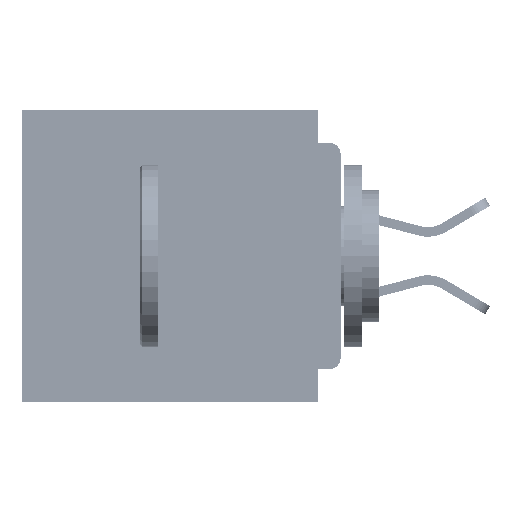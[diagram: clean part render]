
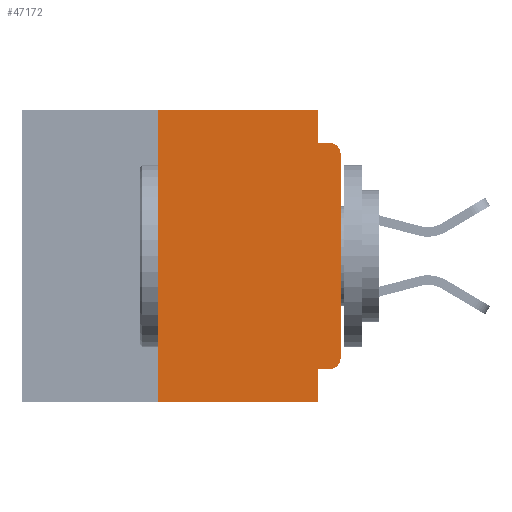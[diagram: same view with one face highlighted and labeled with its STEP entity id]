
A CAD part, left-side view. The second image highlights one B-rep face of the part: STEP entity #47172.
In plain terms, the highlighted planar face has unit normal (-1, 0, 0).
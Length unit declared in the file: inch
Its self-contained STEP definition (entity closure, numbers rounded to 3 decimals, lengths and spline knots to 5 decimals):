
#32 = CARTESIAN_POINT ( 'NONE',  ( 0., 0.25, -0.4 ) ) ;
#1003 = CARTESIAN_POINT ( 'NONE',  ( 0., 0., -0.355 ) ) ;
#1164 = VECTOR ( 'NONE', #13344, 39.37008 ) ;
#1187 = LINE ( 'NONE', #27473, #43794 ) ;
#1316 = CARTESIAN_POINT ( 'NONE',  ( 0., 0.031, 0. ) ) ;
#1366 = DIRECTION ( 'NONE',  ( 0., 0., -1. ) ) ;
#1880 = VECTOR ( 'NONE', #17656, 39.37008 ) ;
#2666 = VECTOR ( 'NONE', #46328, 39.37008 ) ;
#2784 = EDGE_CURVE ( 'NONE', #44498, #15873, #3217, .T. ) ;
#3217 = LINE ( 'NONE', #53201, #23938 ) ;
#3515 = VERTEX_POINT ( 'NONE', #24632 ) ;
#3997 = EDGE_CURVE ( 'NONE', #20755, #44498, #15372, .T. ) ;
#4605 = ORIENTED_EDGE ( 'NONE', *, *, #16691, .T. ) ;
#5073 = DIRECTION ( 'NONE',  ( 0., 0., 1. ) ) ;
#5214 = DIRECTION ( 'NONE',  ( 1., 0., 0. ) ) ;
#5673 = LINE ( 'NONE', #50269, #1164 ) ;
#8948 = CARTESIAN_POINT ( 'NONE',  ( 0., 0.031, -0.045 ) ) ;
#9194 = CARTESIAN_POINT ( 'NONE',  ( 0., 0.015, -0.045 ) ) ;
#9351 = EDGE_CURVE ( 'NONE', #37884, #3515, #34268, .T. ) ;
#9476 = ORIENTED_EDGE ( 'NONE', *, *, #37555, .T. ) ;
#9856 = CIRCLE ( 'NONE', #25262, 0.015 ) ;
#9938 = AXIS2_PLACEMENT_3D ( 'NONE', #29965, #5214, #34076 ) ;
#10541 = EDGE_CURVE ( 'NONE', #29381, #37884, #34785, .T. ) ;
#10884 = ORIENTED_EDGE ( 'NONE', *, *, #32157, .F. ) ;
#13344 = DIRECTION ( 'NONE',  ( 0., 0., 1. ) ) ;
#13378 = PLANE ( 'NONE',  #9938 ) ;
#13827 = LINE ( 'NONE', #25695, #34446 ) ;
#14192 = AXIS2_PLACEMENT_3D ( 'NONE', #47386, #22753, #51515 ) ;
#14402 = LINE ( 'NONE', #30655, #25396 ) ;
#15372 = LINE ( 'NONE', #1316, #46953 ) ;
#15833 = CARTESIAN_POINT ( 'NONE',  ( 0., 0.015, -0.06 ) ) ;
#15873 = VERTEX_POINT ( 'NONE', #9194 ) ;
#16194 = EDGE_LOOP ( 'NONE', ( #9476, #4605, #45202, #19140, #47458, #10884, #35054, #46989, #43441, #47296 ) ) ;
#16691 = EDGE_CURVE ( 'NONE', #48310, #15873, #9856, .T. ) ;
#17656 = DIRECTION ( 'NONE',  ( 0., 1., 0. ) ) ;
#19140 = ORIENTED_EDGE ( 'NONE', *, *, #3997, .F. ) ;
#19234 = CARTESIAN_POINT ( 'NONE',  ( 0., 0.031, 0. ) ) ;
#19500 = EDGE_CURVE ( 'NONE', #33827, #20755, #1187, .T. ) ;
#19990 = DIRECTION ( 'NONE',  ( 0., 0., -1. ) ) ;
#20755 = VERTEX_POINT ( 'NONE', #19234 ) ;
#22753 = DIRECTION ( 'NONE',  ( -1., 0., 0. ) ) ;
#23929 = CIRCLE ( 'NONE', #14192, 0.015 ) ;
#23938 = VECTOR ( 'NONE', #52860, 39.37008 ) ;
#24632 = CARTESIAN_POINT ( 'NONE',  ( 0., 0.031, -0.4 ) ) ;
#25049 = CARTESIAN_POINT ( 'NONE',  ( 0., 0., -0.06 ) ) ;
#25262 = AXIS2_PLACEMENT_3D ( 'NONE', #15833, #44647, #19990 ) ;
#25396 = VECTOR ( 'NONE', #34780, 39.37008 ) ;
#25695 = CARTESIAN_POINT ( 'NONE',  ( 0., 0.25, -0.4 ) ) ;
#27473 = CARTESIAN_POINT ( 'NONE',  ( 0., 0.437, 0. ) ) ;
#28714 = VERTEX_POINT ( 'NONE', #29675 ) ;
#29381 = VERTEX_POINT ( 'NONE', #51012 ) ;
#29675 = CARTESIAN_POINT ( 'NONE',  ( 0., 0., -0.34 ) ) ;
#29965 = CARTESIAN_POINT ( 'NONE',  ( 0., 0.437, 0. ) ) ;
#30100 = CARTESIAN_POINT ( 'NONE',  ( 0., 0.031, -0.4 ) ) ;
#30655 = CARTESIAN_POINT ( 'NONE',  ( 0., 0.437, -0.4 ) ) ;
#32044 = VERTEX_POINT ( 'NONE', #32 ) ;
#32157 = EDGE_CURVE ( 'NONE', #32044, #33827, #13827, .T. ) ;
#32750 = EDGE_CURVE ( 'NONE', #32044, #3515, #14402, .T. ) ;
#33827 = VERTEX_POINT ( 'NONE', #38126 ) ;
#34076 = DIRECTION ( 'NONE',  ( 0., 0., -1. ) ) ;
#34268 = LINE ( 'NONE', #30100, #2666 ) ;
#34446 = VECTOR ( 'NONE', #5073, 39.37008 ) ;
#34780 = DIRECTION ( 'NONE',  ( 0., -1., 0. ) ) ;
#34785 = LINE ( 'NONE', #1003, #1880 ) ;
#35054 = ORIENTED_EDGE ( 'NONE', *, *, #32750, .T. ) ;
#35207 = EDGE_CURVE ( 'NONE', #29381, #28714, #23929, .T. ) ;
#37555 = EDGE_CURVE ( 'NONE', #28714, #48310, #5673, .T. ) ;
#37884 = VERTEX_POINT ( 'NONE', #52202 ) ;
#38126 = CARTESIAN_POINT ( 'NONE',  ( 0., 0.25, 0. ) ) ;
#39877 = DIRECTION ( 'NONE',  ( 0., -1., 0. ) ) ;
#41540 = FACE_OUTER_BOUND ( 'NONE', #16194, .T. ) ;
#43441 = ORIENTED_EDGE ( 'NONE', *, *, #10541, .F. ) ;
#43794 = VECTOR ( 'NONE', #39877, 39.37008 ) ;
#44498 = VERTEX_POINT ( 'NONE', #8948 ) ;
#44647 = DIRECTION ( 'NONE',  ( -1., 0., 0. ) ) ;
#45202 = ORIENTED_EDGE ( 'NONE', *, *, #2784, .F. ) ;
#46328 = DIRECTION ( 'NONE',  ( 0., 0., -1. ) ) ;
#46953 = VECTOR ( 'NONE', #1366, 39.37008 ) ;
#46989 = ORIENTED_EDGE ( 'NONE', *, *, #9351, .F. ) ;
#47172 = ADVANCED_FACE ( 'NONE', ( #41540 ), #13378, .F. ) ;
#47296 = ORIENTED_EDGE ( 'NONE', *, *, #35207, .T. ) ;
#47386 = CARTESIAN_POINT ( 'NONE',  ( 0., 0.015, -0.34 ) ) ;
#47458 = ORIENTED_EDGE ( 'NONE', *, *, #19500, .F. ) ;
#48310 = VERTEX_POINT ( 'NONE', #25049 ) ;
#50269 = CARTESIAN_POINT ( 'NONE',  ( 0., 0., 0. ) ) ;
#51012 = CARTESIAN_POINT ( 'NONE',  ( 0., 0.015, -0.355 ) ) ;
#51515 = DIRECTION ( 'NONE',  ( 0., 0., -1. ) ) ;
#52202 = CARTESIAN_POINT ( 'NONE',  ( 0., 0.031, -0.355 ) ) ;
#52860 = DIRECTION ( 'NONE',  ( 0., -1., 0. ) ) ;
#53201 = CARTESIAN_POINT ( 'NONE',  ( 0., 0., -0.045 ) ) ;
